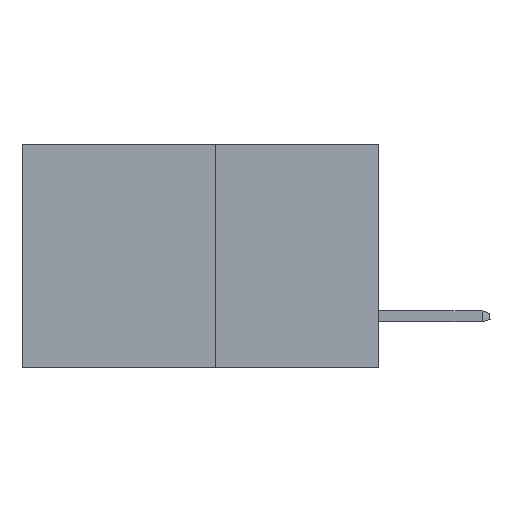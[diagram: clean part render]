
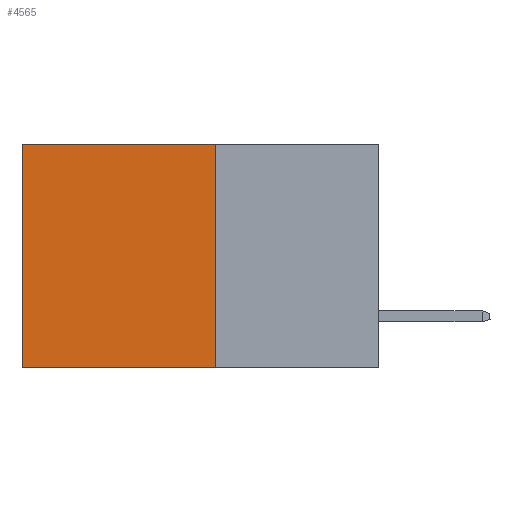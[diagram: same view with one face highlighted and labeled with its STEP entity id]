
A CAD part, left-side view. The second image highlights one B-rep face of the part: STEP entity #4565.
In plain terms, the highlighted planar face has unit normal (-1, 0, 0).
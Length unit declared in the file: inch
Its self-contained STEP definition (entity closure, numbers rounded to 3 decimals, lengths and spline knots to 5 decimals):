
#40 = CARTESIAN_POINT ( 'NONE',  ( 0.277, 0.27, -0.37 ) ) ;
#376 = VECTOR ( 'NONE', #882, 39.37008 ) ;
#882 = DIRECTION ( 'NONE',  ( 0., 1., 0. ) ) ;
#1129 = VERTEX_POINT ( 'NONE', #8045 ) ;
#1230 = PLANE ( 'NONE',  #11644 ) ;
#2241 = EDGE_LOOP ( 'NONE', ( #10106, #6399, #3009, #4446 ) ) ;
#2557 = VERTEX_POINT ( 'NONE', #8757 ) ;
#3009 = ORIENTED_EDGE ( 'NONE', *, *, #10807, .F. ) ;
#3647 = VECTOR ( 'NONE', #5580, 39.37008 ) ;
#3807 = DIRECTION ( 'NONE',  ( 0., 0., -1. ) ) ;
#4446 = ORIENTED_EDGE ( 'NONE', *, *, #7868, .T. ) ;
#4565 = ADVANCED_FACE ( 'NONE', ( #8150 ), #1230, .F. ) ;
#5447 = LINE ( 'NONE', #9248, #10230 ) ;
#5580 = DIRECTION ( 'NONE',  ( 0., 0., -1. ) ) ;
#5660 = VERTEX_POINT ( 'NONE', #6489 ) ;
#6254 = LINE ( 'NONE', #7300, #376 ) ;
#6288 = CARTESIAN_POINT ( 'NONE',  ( 0.277, 0.27, -0.37 ) ) ;
#6399 = ORIENTED_EDGE ( 'NONE', *, *, #10688, .F. ) ;
#6489 = CARTESIAN_POINT ( 'NONE',  ( 0.277, 0.59, 0. ) ) ;
#6495 = DIRECTION ( 'NONE',  ( 0., 0., -1. ) ) ;
#6907 = VECTOR ( 'NONE', #8074, 39.37008 ) ;
#7300 = CARTESIAN_POINT ( 'NONE',  ( 0.277, 0.27, 0. ) ) ;
#7868 = EDGE_CURVE ( 'NONE', #8571, #5660, #6254, .T. ) ;
#8045 = CARTESIAN_POINT ( 'NONE',  ( 0.277, 0.59, -0.37 ) ) ;
#8074 = DIRECTION ( 'NONE',  ( 0., 1., 0. ) ) ;
#8150 = FACE_OUTER_BOUND ( 'NONE', #2241, .T. ) ;
#8571 = VERTEX_POINT ( 'NONE', #10800 ) ;
#8757 = CARTESIAN_POINT ( 'NONE',  ( 0.277, 0.27, -0.37 ) ) ;
#9244 = LINE ( 'NONE', #6288, #6907 ) ;
#9248 = CARTESIAN_POINT ( 'NONE',  ( 0.277, 0.59, -0.37 ) ) ;
#10063 = CARTESIAN_POINT ( 'NONE',  ( 0.277, 0.27, -0.37 ) ) ;
#10106 = ORIENTED_EDGE ( 'NONE', *, *, #11480, .T. ) ;
#10230 = VECTOR ( 'NONE', #3807, 39.37008 ) ;
#10407 = DIRECTION ( 'NONE',  ( 1., 0., 0. ) ) ;
#10688 = EDGE_CURVE ( 'NONE', #2557, #1129, #9244, .T. ) ;
#10800 = CARTESIAN_POINT ( 'NONE',  ( 0.277, 0.27, 0. ) ) ;
#10807 = EDGE_CURVE ( 'NONE', #8571, #2557, #11217, .T. ) ;
#11217 = LINE ( 'NONE', #10063, #3647 ) ;
#11480 = EDGE_CURVE ( 'NONE', #5660, #1129, #5447, .T. ) ;
#11644 = AXIS2_PLACEMENT_3D ( 'NONE', #40, #10407, #6495 ) ;
